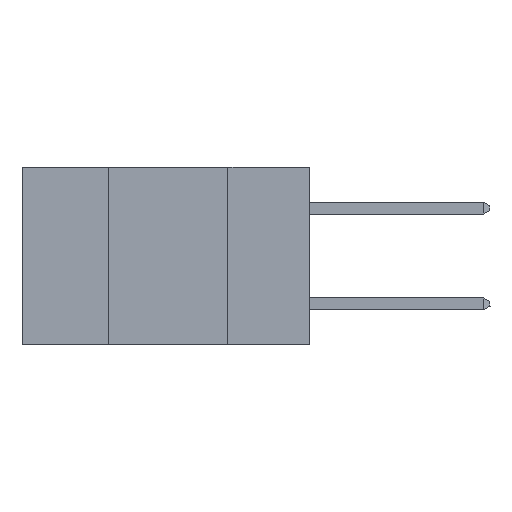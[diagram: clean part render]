
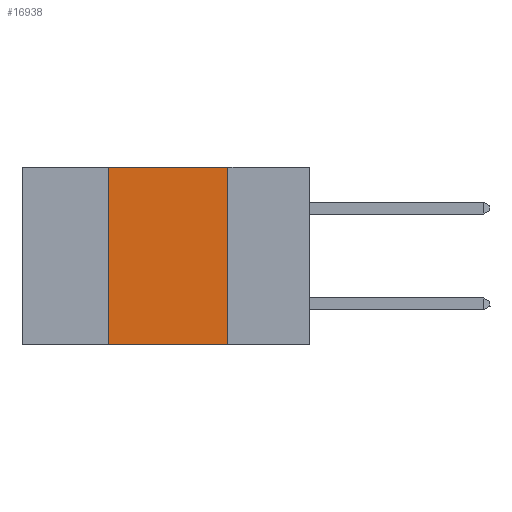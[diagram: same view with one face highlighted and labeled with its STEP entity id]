
A CAD part, left-side view. The second image highlights one B-rep face of the part: STEP entity #16938.
In plain terms, the highlighted planar face has unit normal (-1, 0, 0).
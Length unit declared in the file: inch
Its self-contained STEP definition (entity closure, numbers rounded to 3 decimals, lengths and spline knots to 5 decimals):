
#3 = CARTESIAN_POINT ( 'NONE',  ( 0., 0.6, 0. ) ) ;
#490 = EDGE_CURVE ( 'NONE', #14291, #11073, #18942, .T. ) ;
#1360 = LINE ( 'NONE', #20702, #18881 ) ;
#1751 = CARTESIAN_POINT ( 'NONE',  ( 0., 0.17, 0. ) ) ;
#2316 = DIRECTION ( 'NONE',  ( 0., 0., -1. ) ) ;
#2400 = EDGE_CURVE ( 'NONE', #15869, #14291, #19095, .T. ) ;
#5721 = PLANE ( 'NONE',  #17938 ) ;
#6232 = VERTEX_POINT ( 'NONE', #9184 ) ;
#6626 = LINE ( 'NONE', #1751, #7232 ) ;
#7232 = VECTOR ( 'NONE', #2316, 39.37008 ) ;
#8418 = FACE_OUTER_BOUND ( 'NONE', #15108, .T. ) ;
#9184 = CARTESIAN_POINT ( 'NONE',  ( 0., 0.17, -0.37 ) ) ;
#11073 = VERTEX_POINT ( 'NONE', #20911 ) ;
#13051 = CARTESIAN_POINT ( 'NONE',  ( 0., 0.42, 0. ) ) ;
#14291 = VERTEX_POINT ( 'NONE', #26354 ) ;
#14868 = CARTESIAN_POINT ( 'NONE',  ( 0., 0.6, 0. ) ) ;
#15108 = EDGE_LOOP ( 'NONE', ( #27229, #24444, #19207, #23742 ) ) ;
#15869 = VERTEX_POINT ( 'NONE', #17915 ) ;
#16938 = ADVANCED_FACE ( 'NONE', ( #8418 ), #5721, .F. ) ;
#17125 = DIRECTION ( 'NONE',  ( 0., 0., 1. ) ) ;
#17915 = CARTESIAN_POINT ( 'NONE',  ( 0., 0.42, -0.37 ) ) ;
#17938 = AXIS2_PLACEMENT_3D ( 'NONE', #14868, #27319, #23371 ) ;
#18881 = VECTOR ( 'NONE', #22523, 39.37008 ) ;
#18942 = LINE ( 'NONE', #3, #25231 ) ;
#19095 = LINE ( 'NONE', #13051, #19789 ) ;
#19207 = ORIENTED_EDGE ( 'NONE', *, *, #2400, .F. ) ;
#19789 = VECTOR ( 'NONE', #17125, 39.37008 ) ;
#20702 = CARTESIAN_POINT ( 'NONE',  ( 0., 0.6, -0.37 ) ) ;
#20911 = CARTESIAN_POINT ( 'NONE',  ( 0., 0.17, 0. ) ) ;
#22523 = DIRECTION ( 'NONE',  ( 0., -1., 0. ) ) ;
#23257 = DIRECTION ( 'NONE',  ( 0., -1., 0. ) ) ;
#23371 = DIRECTION ( 'NONE',  ( 0., 0., -1. ) ) ;
#23742 = ORIENTED_EDGE ( 'NONE', *, *, #24683, .T. ) ;
#24444 = ORIENTED_EDGE ( 'NONE', *, *, #490, .F. ) ;
#24683 = EDGE_CURVE ( 'NONE', #15869, #6232, #1360, .T. ) ;
#25231 = VECTOR ( 'NONE', #23257, 39.37008 ) ;
#26354 = CARTESIAN_POINT ( 'NONE',  ( 0., 0.42, 0. ) ) ;
#26550 = EDGE_CURVE ( 'NONE', #11073, #6232, #6626, .T. ) ;
#27229 = ORIENTED_EDGE ( 'NONE', *, *, #26550, .F. ) ;
#27319 = DIRECTION ( 'NONE',  ( 1., 0., 0. ) ) ;
